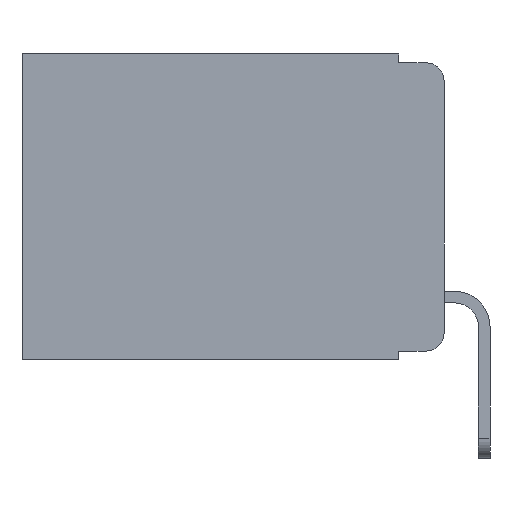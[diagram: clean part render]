
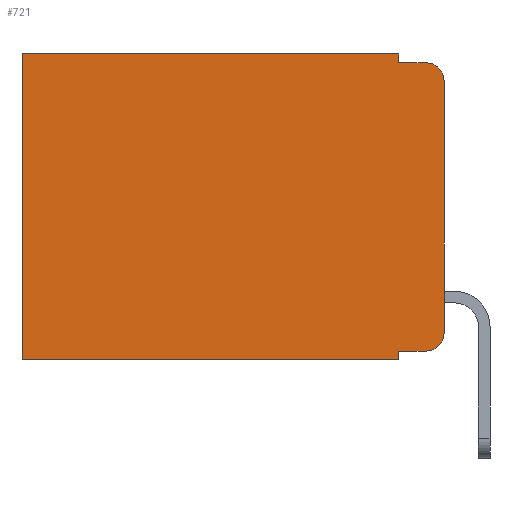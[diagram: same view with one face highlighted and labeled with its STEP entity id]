
A CAD part, left-side view. The second image highlights one B-rep face of the part: STEP entity #721.
In plain terms, the highlighted planar face has unit normal (-1, 0, 0).
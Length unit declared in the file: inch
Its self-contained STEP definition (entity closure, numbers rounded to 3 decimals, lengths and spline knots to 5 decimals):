
#133 = VECTOR ( 'NONE', #644, 39.37008 ) ;
#310 = VERTEX_POINT ( 'NONE', #3428 ) ;
#453 = LINE ( 'NONE', #6940, #12518 ) ;
#472 = VECTOR ( 'NONE', #1190, 39.37008 ) ;
#580 = DIRECTION ( 'NONE',  ( 0., 0., -1. ) ) ;
#644 = DIRECTION ( 'NONE',  ( 0., -1., 0. ) ) ;
#704 = DIRECTION ( 'NONE',  ( -1., 0., 0. ) ) ;
#721 = ADVANCED_FACE ( 'NONE', ( #12870 ), #12910, .F. ) ;
#843 = CARTESIAN_POINT ( 'NONE',  ( 0.298, 0., -0.03 ) ) ;
#868 = VECTOR ( 'NONE', #10303, 39.37008 ) ;
#1190 = DIRECTION ( 'NONE',  ( 0., 1., 0. ) ) ;
#1329 = VERTEX_POINT ( 'NONE', #5934 ) ;
#1687 = CIRCLE ( 'NONE', #9948, 0.02 ) ;
#1925 = DIRECTION ( 'NONE',  ( 1., 0., 0. ) ) ;
#1930 = CARTESIAN_POINT ( 'NONE',  ( 0.298, 0.473, 0. ) ) ;
#3127 = CARTESIAN_POINT ( 'NONE',  ( 0.298, 0., 0. ) ) ;
#3428 = CARTESIAN_POINT ( 'NONE',  ( 0.298, 0., -0.313 ) ) ;
#3955 = VECTOR ( 'NONE', #8090, 39.37008 ) ;
#4165 = CARTESIAN_POINT ( 'NONE',  ( 0.298, 0.473, 0. ) ) ;
#4344 = LINE ( 'NONE', #14106, #10209 ) ;
#4861 = EDGE_LOOP ( 'NONE', ( #8419, #8561, #8577, #8688, #8700, #8860, #8988, #9036, #9052, #9218 ) ) ;
#5640 = CARTESIAN_POINT ( 'NONE',  ( 0.298, 0.051, -0.01 ) ) ;
#5696 = DIRECTION ( 'NONE',  ( -1., 0., 0. ) ) ;
#5934 = CARTESIAN_POINT ( 'NONE',  ( 0.298, 0.02, -0.01 ) ) ;
#6100 = VERTEX_POINT ( 'NONE', #13703 ) ;
#6843 = DIRECTION ( 'NONE',  ( 0., 0., -1. ) ) ;
#6940 = CARTESIAN_POINT ( 'NONE',  ( 0.298, 0.051, 0. ) ) ;
#7154 = CARTESIAN_POINT ( 'NONE',  ( 0.298, 0.473, -0.343 ) ) ;
#7412 = VERTEX_POINT ( 'NONE', #13412 ) ;
#7544 = LINE ( 'NONE', #5640, #868 ) ;
#7565 = LINE ( 'NONE', #12729, #472 ) ;
#7760 = CARTESIAN_POINT ( 'NONE',  ( 0.298, 0., 0. ) ) ;
#7927 = LINE ( 'NONE', #3127, #10849 ) ;
#8027 = VERTEX_POINT ( 'NONE', #4165 ) ;
#8090 = DIRECTION ( 'NONE',  ( 0., 0., -1. ) ) ;
#8191 = CARTESIAN_POINT ( 'NONE',  ( 0.298, 0.02, -0.313 ) ) ;
#8291 = EDGE_CURVE ( 'NONE', #12171, #8027, #13298, .T. ) ;
#8419 = ORIENTED_EDGE ( 'NONE', *, *, #9497, .F. ) ;
#8561 = ORIENTED_EDGE ( 'NONE', *, *, #9516, .T. ) ;
#8577 = ORIENTED_EDGE ( 'NONE', *, *, #9518, .F. ) ;
#8688 = ORIENTED_EDGE ( 'NONE', *, *, #9521, .F. ) ;
#8700 = ORIENTED_EDGE ( 'NONE', *, *, #8291, .T. ) ;
#8860 = ORIENTED_EDGE ( 'NONE', *, *, #9543, .T. ) ;
#8988 = ORIENTED_EDGE ( 'NONE', *, *, #9264, .F. ) ;
#9036 = ORIENTED_EDGE ( 'NONE', *, *, #9547, .F. ) ;
#9052 = ORIENTED_EDGE ( 'NONE', *, *, #9549, .T. ) ;
#9218 = ORIENTED_EDGE ( 'NONE', *, *, #9570, .T. ) ;
#9264 = EDGE_CURVE ( 'NONE', #9372, #11810, #7565, .T. ) ;
#9347 = DIRECTION ( 'NONE',  ( 0., 0., -1. ) ) ;
#9372 = VERTEX_POINT ( 'NONE', #11988 ) ;
#9494 = CARTESIAN_POINT ( 'NONE',  ( 0.298, 0., 0. ) ) ;
#9497 = EDGE_CURVE ( 'NONE', #10820, #310, #7927, .T. ) ;
#9516 = EDGE_CURVE ( 'NONE', #10820, #1329, #1687, .T. ) ;
#9518 = EDGE_CURVE ( 'NONE', #6100, #1329, #7544, .T. ) ;
#9521 = EDGE_CURVE ( 'NONE', #12171, #6100, #4344, .T. ) ;
#9543 = EDGE_CURVE ( 'NONE', #8027, #11810, #13124, .T. ) ;
#9547 = EDGE_CURVE ( 'NONE', #7412, #9372, #453, .T. ) ;
#9549 = EDGE_CURVE ( 'NONE', #7412, #13900, #9883, .T. ) ;
#9570 = EDGE_CURVE ( 'NONE', #13900, #310, #12837, .T. ) ;
#9883 = LINE ( 'NONE', #11355, #133 ) ;
#9948 = AXIS2_PLACEMENT_3D ( 'NONE', #12283, #5696, #13223 ) ;
#10209 = VECTOR ( 'NONE', #580, 39.37008 ) ;
#10303 = DIRECTION ( 'NONE',  ( 0., -1., 0. ) ) ;
#10646 = AXIS2_PLACEMENT_3D ( 'NONE', #8191, #704, #9347 ) ;
#10756 = VECTOR ( 'NONE', #14335, 39.37008 ) ;
#10820 = VERTEX_POINT ( 'NONE', #843 ) ;
#10849 = VECTOR ( 'NONE', #6843, 39.37008 ) ;
#11333 = CARTESIAN_POINT ( 'NONE',  ( 0.298, 0.02, -0.333 ) ) ;
#11355 = CARTESIAN_POINT ( 'NONE',  ( 0.298, 0.051, -0.333 ) ) ;
#11810 = VERTEX_POINT ( 'NONE', #7154 ) ;
#11846 = CARTESIAN_POINT ( 'NONE',  ( 0.298, 0.051, 0. ) ) ;
#11988 = CARTESIAN_POINT ( 'NONE',  ( 0.298, 0.051, -0.343 ) ) ;
#12171 = VERTEX_POINT ( 'NONE', #11846 ) ;
#12283 = CARTESIAN_POINT ( 'NONE',  ( 0.298, 0.02, -0.03 ) ) ;
#12518 = VECTOR ( 'NONE', #14145, 39.37008 ) ;
#12729 = CARTESIAN_POINT ( 'NONE',  ( 0.298, 0., -0.343 ) ) ;
#12837 = CIRCLE ( 'NONE', #10646, 0.02 ) ;
#12870 = FACE_OUTER_BOUND ( 'NONE', #4861, .T. ) ;
#12910 = PLANE ( 'NONE',  #14519 ) ;
#13124 = LINE ( 'NONE', #1930, #3955 ) ;
#13223 = DIRECTION ( 'NONE',  ( 0., 0., -1. ) ) ;
#13298 = LINE ( 'NONE', #9494, #10756 ) ;
#13412 = CARTESIAN_POINT ( 'NONE',  ( 0.298, 0.051, -0.333 ) ) ;
#13649 = DIRECTION ( 'NONE',  ( 0., 0., -1. ) ) ;
#13703 = CARTESIAN_POINT ( 'NONE',  ( 0.298, 0.051, -0.01 ) ) ;
#13900 = VERTEX_POINT ( 'NONE', #11333 ) ;
#14106 = CARTESIAN_POINT ( 'NONE',  ( 0.298, 0.051, 0. ) ) ;
#14145 = DIRECTION ( 'NONE',  ( 0., 0., -1. ) ) ;
#14335 = DIRECTION ( 'NONE',  ( 0., 1., 0. ) ) ;
#14519 = AXIS2_PLACEMENT_3D ( 'NONE', #7760, #1925, #13649 ) ;
